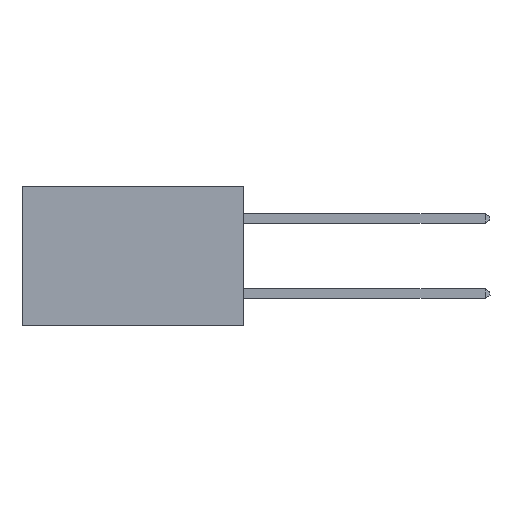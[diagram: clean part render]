
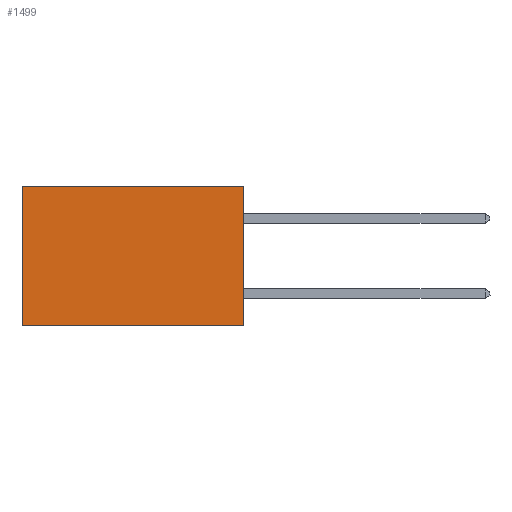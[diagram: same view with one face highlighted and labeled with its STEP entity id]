
A CAD part, left-side view. The second image highlights one B-rep face of the part: STEP entity #1499.
In plain terms, the highlighted planar face has unit normal (-1, 0, 0).
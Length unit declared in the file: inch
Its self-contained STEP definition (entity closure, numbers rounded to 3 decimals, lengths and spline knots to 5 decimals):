
#86 = VERTEX_POINT ( 'NONE', #8095 ) ;
#1186 = ORIENTED_EDGE ( 'NONE', *, *, #2306, .T. ) ;
#1314 = CARTESIAN_POINT ( 'NONE',  ( 0.277, 0.59, -0.37 ) ) ;
#1326 = DIRECTION ( 'NONE',  ( 0., 0., -1. ) ) ;
#1479 = CARTESIAN_POINT ( 'NONE',  ( 0.277, 0., -0.37 ) ) ;
#1499 = ADVANCED_FACE ( 'NONE', ( #3976 ), #5021, .F. ) ;
#1934 = CARTESIAN_POINT ( 'NONE',  ( 0.277, 0., 0. ) ) ;
#2306 = EDGE_CURVE ( 'NONE', #6810, #8179, #8772, .T. ) ;
#2320 = VECTOR ( 'NONE', #7070, 39.37008 ) ;
#2328 = VECTOR ( 'NONE', #2824, 39.37008 ) ;
#2566 = CARTESIAN_POINT ( 'NONE',  ( 0.277, 0., 0. ) ) ;
#2824 = DIRECTION ( 'NONE',  ( 0., 0., -1. ) ) ;
#2904 = ORIENTED_EDGE ( 'NONE', *, *, #7567, .T. ) ;
#3556 = DIRECTION ( 'NONE',  ( 1., 0., 0. ) ) ;
#3773 = CARTESIAN_POINT ( 'NONE',  ( 0.277, 0., -0.37 ) ) ;
#3976 = FACE_OUTER_BOUND ( 'NONE', #4269, .T. ) ;
#4269 = EDGE_LOOP ( 'NONE', ( #2904, #4859, #8765, #1186 ) ) ;
#4270 = LINE ( 'NONE', #7605, #2320 ) ;
#4859 = ORIENTED_EDGE ( 'NONE', *, *, #6562, .F. ) ;
#5021 = PLANE ( 'NONE',  #6604 ) ;
#5818 = VECTOR ( 'NONE', #1326, 39.37008 ) ;
#5847 = DIRECTION ( 'NONE',  ( 0., 0., -1. ) ) ;
#6112 = EDGE_CURVE ( 'NONE', #6810, #8271, #6433, .T. ) ;
#6433 = LINE ( 'NONE', #3773, #2328 ) ;
#6562 = EDGE_CURVE ( 'NONE', #8271, #86, #4270, .T. ) ;
#6604 = AXIS2_PLACEMENT_3D ( 'NONE', #1479, #3556, #5847 ) ;
#6810 = VERTEX_POINT ( 'NONE', #2566 ) ;
#7070 = DIRECTION ( 'NONE',  ( 0., 1., 0. ) ) ;
#7091 = CARTESIAN_POINT ( 'NONE',  ( 0.277, 0., -0.37 ) ) ;
#7381 = CARTESIAN_POINT ( 'NONE',  ( 0.277, 0.59, 0. ) ) ;
#7567 = EDGE_CURVE ( 'NONE', #8179, #86, #7600, .T. ) ;
#7600 = LINE ( 'NONE', #1314, #5818 ) ;
#7605 = CARTESIAN_POINT ( 'NONE',  ( 0.277, 0., -0.37 ) ) ;
#7881 = DIRECTION ( 'NONE',  ( 0., 1., 0. ) ) ;
#8095 = CARTESIAN_POINT ( 'NONE',  ( 0.277, 0.59, -0.37 ) ) ;
#8179 = VERTEX_POINT ( 'NONE', #7381 ) ;
#8271 = VERTEX_POINT ( 'NONE', #7091 ) ;
#8325 = VECTOR ( 'NONE', #7881, 39.37008 ) ;
#8765 = ORIENTED_EDGE ( 'NONE', *, *, #6112, .F. ) ;
#8772 = LINE ( 'NONE', #1934, #8325 ) ;
